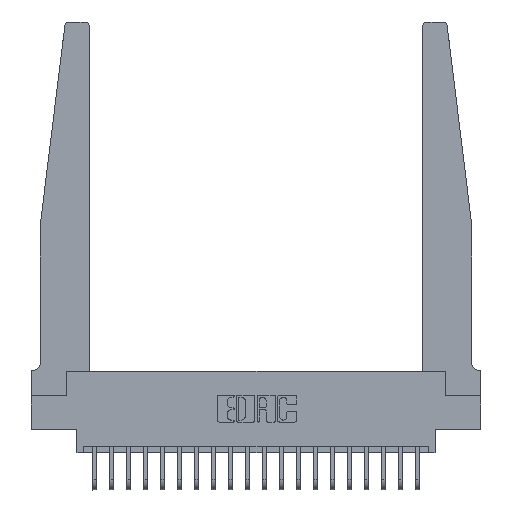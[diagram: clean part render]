
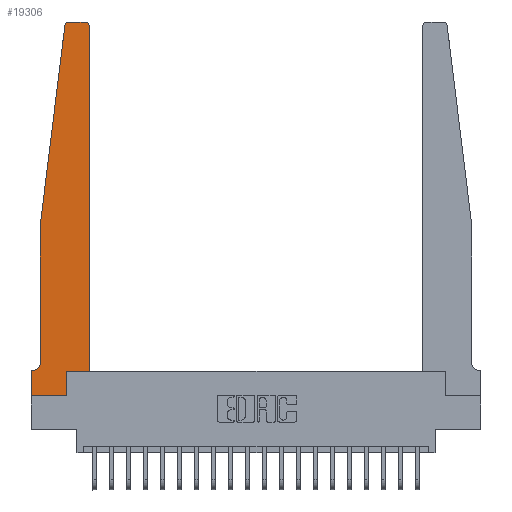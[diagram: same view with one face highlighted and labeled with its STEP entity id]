
A CAD part, top view. The second image highlights one B-rep face of the part: STEP entity #19306.
In plain terms, the highlighted planar face has unit normal (0, 0, 1).
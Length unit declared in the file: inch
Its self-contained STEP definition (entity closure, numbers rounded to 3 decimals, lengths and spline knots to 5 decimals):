
#441 = CARTESIAN_POINT ( 'NONE',  ( 0.425, 2.72, 0.37 ) ) ;
#679 = EDGE_CURVE ( 'NONE', #13821, #3755, #12768, .T. ) ;
#803 = EDGE_CURVE ( 'NONE', #13668, #13821, #11779, .T. ) ;
#895 = CARTESIAN_POINT ( 'NONE',  ( 0.065, 1.25, 0.37 ) ) ;
#1042 = LINE ( 'NONE', #16928, #9007 ) ;
#1182 = EDGE_CURVE ( 'NONE', #6977, #8997, #12256, .T. ) ;
#1185 = CARTESIAN_POINT ( 'NONE',  ( 0.065, 0.2375, 0.37 ) ) ;
#1234 = VECTOR ( 'NONE', #11743, 39.37008 ) ;
#1474 = EDGE_CURVE ( 'NONE', #2161, #10422, #16157, .T. ) ;
#1645 = LINE ( 'NONE', #9733, #5872 ) ;
#1916 = DIRECTION ( 'NONE',  ( 0., 0., -1. ) ) ;
#2161 = VERTEX_POINT ( 'NONE', #10766 ) ;
#2623 = DIRECTION ( 'NONE',  ( -1., 0., 0. ) ) ;
#2625 = CARTESIAN_POINT ( 'NONE',  ( 0.015, 0.1875, 0.37 ) ) ;
#2901 = CARTESIAN_POINT ( 'NONE',  ( 0.395, 2.75, 0.37 ) ) ;
#3039 = DIRECTION ( 'NONE',  ( 0., 0., 1. ) ) ;
#3230 = EDGE_CURVE ( 'NONE', #10422, #18798, #5967, .T. ) ;
#3755 = VERTEX_POINT ( 'NONE', #14650 ) ;
#3914 = VECTOR ( 'NONE', #11398, 39.37008 ) ;
#4155 = VECTOR ( 'NONE', #5696, 39.37008 ) ;
#4706 = DIRECTION ( 'NONE',  ( 1., 0., 0. ) ) ;
#5440 = CARTESIAN_POINT ( 'NONE',  ( 0.065, 1.25, 0.37 ) ) ;
#5503 = VERTEX_POINT ( 'NONE', #11351 ) ;
#5696 = DIRECTION ( 'NONE',  ( -0.122, -0.992, 0. ) ) ;
#5764 = CARTESIAN_POINT ( 'NONE',  ( 0., 0., 0.37 ) ) ;
#5782 = VERTEX_POINT ( 'NONE', #2625 ) ;
#5872 = VECTOR ( 'NONE', #11220, 39.37008 ) ;
#5967 = LINE ( 'NONE', #5440, #1234 ) ;
#6237 = AXIS2_PLACEMENT_3D ( 'NONE', #12442, #3039, #14010 ) ;
#6405 = CIRCLE ( 'NONE', #19916, 0.05 ) ;
#6977 = VERTEX_POINT ( 'NONE', #17865 ) ;
#6995 = DIRECTION ( 'NONE',  ( -1., 0., 0. ) ) ;
#7264 = FACE_OUTER_BOUND ( 'NONE', #12036, .T. ) ;
#7364 = DIRECTION ( 'NONE',  ( 1., 0., 0. ) ) ;
#7365 = DIRECTION ( 'NONE',  ( 0., 0., 1. ) ) ;
#7495 = CARTESIAN_POINT ( 'NONE',  ( 0., 0.1875, 0.37 ) ) ;
#7526 = CARTESIAN_POINT ( 'NONE',  ( 0.425, 0.18, 0.37 ) ) ;
#8301 = VECTOR ( 'NONE', #2623, 39.37008 ) ;
#8435 = CIRCLE ( 'NONE', #16907, 0.03 ) ;
#8628 = VECTOR ( 'NONE', #4706, 39.37008 ) ;
#8742 = ORIENTED_EDGE ( 'NONE', *, *, #1182, .T. ) ;
#8997 = VERTEX_POINT ( 'NONE', #7526 ) ;
#9007 = VECTOR ( 'NONE', #9153, 39.37008 ) ;
#9153 = DIRECTION ( 'NONE',  ( 0., 1., 0. ) ) ;
#9618 = CARTESIAN_POINT ( 'NONE',  ( 0., 0., 0.37 ) ) ;
#9628 = ORIENTED_EDGE ( 'NONE', *, *, #14638, .T. ) ;
#9733 = CARTESIAN_POINT ( 'NONE',  ( 0.425, 0.18, 0.37 ) ) ;
#9740 = ORIENTED_EDGE ( 'NONE', *, *, #679, .T. ) ;
#10113 = CARTESIAN_POINT ( 'NONE',  ( 0.25, 2.75, 0.37 ) ) ;
#10345 = VECTOR ( 'NONE', #10569, 39.37008 ) ;
#10422 = VERTEX_POINT ( 'NONE', #16152 ) ;
#10569 = DIRECTION ( 'NONE',  ( 0., -1., 0. ) ) ;
#10766 = CARTESIAN_POINT ( 'NONE',  ( 0.24675, 2.72367, 0.37 ) ) ;
#10956 = CIRCLE ( 'NONE', #6237, 0.03 ) ;
#10983 = VERTEX_POINT ( 'NONE', #441 ) ;
#11113 = EDGE_CURVE ( 'NONE', #5782, #13668, #16097, .T. ) ;
#11220 = DIRECTION ( 'NONE',  ( 0., 1., 0. ) ) ;
#11351 = CARTESIAN_POINT ( 'NONE',  ( 0.27653, 2.75, 0.37 ) ) ;
#11353 = CARTESIAN_POINT ( 'NONE',  ( 0.015, 0.2375, 0.37 ) ) ;
#11398 = DIRECTION ( 'NONE',  ( 1., 0., 0. ) ) ;
#11743 = DIRECTION ( 'NONE',  ( 0., -1., 0. ) ) ;
#11773 = EDGE_CURVE ( 'NONE', #3755, #6977, #1042, .T. ) ;
#11779 = LINE ( 'NONE', #9618, #10345 ) ;
#12008 = PLANE ( 'NONE',  #19486 ) ;
#12024 = CARTESIAN_POINT ( 'NONE',  ( 0.065, 0.1875, 0.37 ) ) ;
#12036 = EDGE_LOOP ( 'NONE', ( #17621, #17659, #13312, #18721, #9628, #12881, #12752, #9740, #13252, #8742, #19794, #20136 ) ) ;
#12256 = LINE ( 'NONE', #12980, #3914 ) ;
#12442 = CARTESIAN_POINT ( 'NONE',  ( 0.27653, 2.72, 0.37 ) ) ;
#12491 = CARTESIAN_POINT ( 'NONE',  ( 0., 0., 0.37 ) ) ;
#12752 = ORIENTED_EDGE ( 'NONE', *, *, #803, .T. ) ;
#12768 = LINE ( 'NONE', #5764, #8628 ) ;
#12881 = ORIENTED_EDGE ( 'NONE', *, *, #11113, .T. ) ;
#12929 = DIRECTION ( 'NONE',  ( -1., 0., 0. ) ) ;
#12980 = CARTESIAN_POINT ( 'NONE',  ( 0.425, 0.18, 0.37 ) ) ;
#13252 = ORIENTED_EDGE ( 'NONE', *, *, #11773, .T. ) ;
#13312 = ORIENTED_EDGE ( 'NONE', *, *, #1474, .T. ) ;
#13607 = EDGE_CURVE ( 'NONE', #10983, #14955, #8435, .T. ) ;
#13668 = VERTEX_POINT ( 'NONE', #7495 ) ;
#13821 = VERTEX_POINT ( 'NONE', #12491 ) ;
#14010 = DIRECTION ( 'NONE',  ( 1., 0., 0. ) ) ;
#14135 = EDGE_CURVE ( 'NONE', #14955, #5503, #19888, .T. ) ;
#14638 = EDGE_CURVE ( 'NONE', #18798, #5782, #6405, .T. ) ;
#14650 = CARTESIAN_POINT ( 'NONE',  ( 0.2605, 0., 0.37 ) ) ;
#14955 = VERTEX_POINT ( 'NONE', #2901 ) ;
#15721 = VECTOR ( 'NONE', #6995, 39.37008 ) ;
#16097 = LINE ( 'NONE', #12024, #8301 ) ;
#16152 = CARTESIAN_POINT ( 'NONE',  ( 0.065, 1.25, 0.37 ) ) ;
#16157 = LINE ( 'NONE', #895, #4155 ) ;
#16361 = EDGE_CURVE ( 'NONE', #8997, #10983, #1645, .T. ) ;
#16742 = DIRECTION ( 'NONE',  ( 0., 0., 1. ) ) ;
#16743 = CARTESIAN_POINT ( 'NONE',  ( 0.395, 2.72, 0.37 ) ) ;
#16907 = AXIS2_PLACEMENT_3D ( 'NONE', #16743, #7365, #18303 ) ;
#16928 = CARTESIAN_POINT ( 'NONE',  ( 0.2605, 0.18, 0.37 ) ) ;
#17621 = ORIENTED_EDGE ( 'NONE', *, *, #14135, .T. ) ;
#17659 = ORIENTED_EDGE ( 'NONE', *, *, #18846, .T. ) ;
#17865 = CARTESIAN_POINT ( 'NONE',  ( 0.2605, 0.18, 0.37 ) ) ;
#18303 = DIRECTION ( 'NONE',  ( 1., 0., 0. ) ) ;
#18721 = ORIENTED_EDGE ( 'NONE', *, *, #3230, .T. ) ;
#18798 = VERTEX_POINT ( 'NONE', #1185 ) ;
#18846 = EDGE_CURVE ( 'NONE', #5503, #2161, #10956, .T. ) ;
#19306 = ADVANCED_FACE ( 'NONE', ( #7264 ), #12008, .T. ) ;
#19486 = AXIS2_PLACEMENT_3D ( 'NONE', #19804, #16742, #7364 ) ;
#19794 = ORIENTED_EDGE ( 'NONE', *, *, #16361, .T. ) ;
#19804 = CARTESIAN_POINT ( 'NONE',  ( 0., 0.1875, 0.37 ) ) ;
#19888 = LINE ( 'NONE', #10113, #15721 ) ;
#19916 = AXIS2_PLACEMENT_3D ( 'NONE', #11353, #1916, #12929 ) ;
#20136 = ORIENTED_EDGE ( 'NONE', *, *, #13607, .T. ) ;
